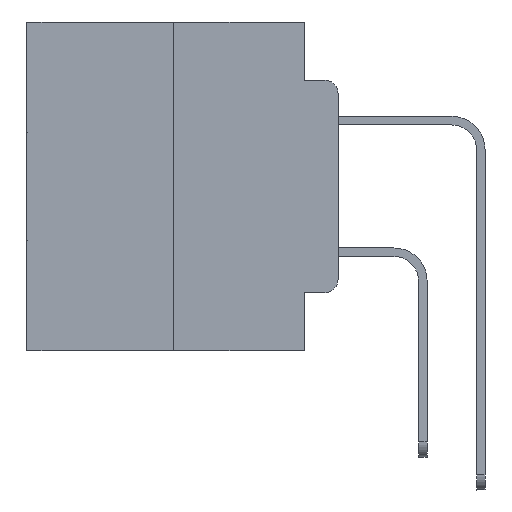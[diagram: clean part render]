
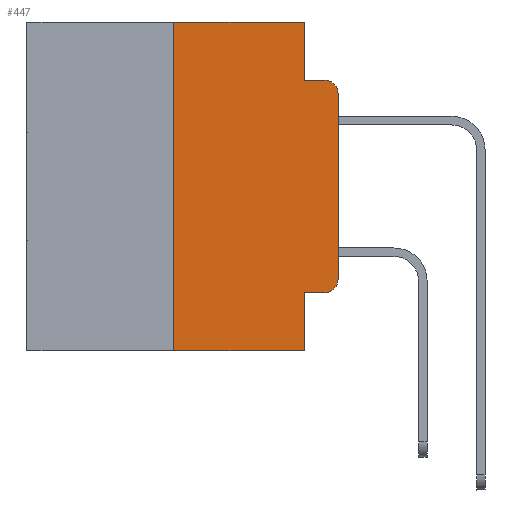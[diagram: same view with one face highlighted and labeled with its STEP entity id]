
A CAD part, left-side view. The second image highlights one B-rep face of the part: STEP entity #447.
In plain terms, the highlighted planar face has unit normal (-1, 0, 0).
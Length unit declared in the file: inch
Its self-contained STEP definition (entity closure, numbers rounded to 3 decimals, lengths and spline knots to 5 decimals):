
#235 = EDGE_CURVE ( 'NONE', #19456, #12653, #22471, .T. ) ;
#362 = VECTOR ( 'NONE', #22300, 39.37008 ) ;
#447 = ADVANCED_FACE ( 'NONE', ( #14925 ), #15079, .F. ) ;
#984 = CARTESIAN_POINT ( 'NONE',  ( 0., 0.02, -0.3915 ) ) ;
#1323 = DIRECTION ( 'NONE',  ( -1., 0., 0. ) ) ;
#1924 = CARTESIAN_POINT ( 'NONE',  ( 0., 0., 0. ) ) ;
#1973 = DIRECTION ( 'NONE',  ( 0., -1., 0. ) ) ;
#2966 = CARTESIAN_POINT ( 'NONE',  ( 0., 0., -0.1085 ) ) ;
#3199 = DIRECTION ( 'NONE',  ( 0., 0., -1. ) ) ;
#3231 = EDGE_CURVE ( 'NONE', #5641, #22865, #3987, .T. ) ;
#3450 = VECTOR ( 'NONE', #3199, 39.37008 ) ;
#3684 = CARTESIAN_POINT ( 'NONE',  ( 0., 0.473, 0. ) ) ;
#3987 = LINE ( 'NONE', #13137, #362 ) ;
#4691 = VECTOR ( 'NONE', #29355, 39.37008 ) ;
#5473 = DIRECTION ( 'NONE',  ( 0., 0., -1. ) ) ;
#5543 = VECTOR ( 'NONE', #1973, 39.37008 ) ;
#5582 = AXIS2_PLACEMENT_3D ( 'NONE', #3684, #28126, #5933 ) ;
#5641 = VERTEX_POINT ( 'NONE', #26946 ) ;
#5727 = CARTESIAN_POINT ( 'NONE',  ( 0., 0.051, -0.0885 ) ) ;
#5933 = DIRECTION ( 'NONE',  ( 0., 0., -1. ) ) ;
#6357 = EDGE_LOOP ( 'NONE', ( #26789, #13331, #10623, #20446, #7698, #7460, #16850, #11954, #8462, #14721 ) ) ;
#6523 = VERTEX_POINT ( 'NONE', #20113 ) ;
#6768 = CIRCLE ( 'NONE', #25910, 0.02 ) ;
#6802 = EDGE_CURVE ( 'NONE', #23607, #6523, #17517, .T. ) ;
#7460 = ORIENTED_EDGE ( 'NONE', *, *, #8773, .F. ) ;
#7513 = CARTESIAN_POINT ( 'NONE',  ( 0., 0., -0.3915 ) ) ;
#7698 = ORIENTED_EDGE ( 'NONE', *, *, #21882, .F. ) ;
#8462 = ORIENTED_EDGE ( 'NONE', *, *, #22431, .T. ) ;
#8677 = CARTESIAN_POINT ( 'NONE',  ( 0., 0.051, -0.5 ) ) ;
#8703 = CARTESIAN_POINT ( 'NONE',  ( 0., 0.051, 0. ) ) ;
#8773 = EDGE_CURVE ( 'NONE', #5641, #13053, #28066, .T. ) ;
#8886 = CARTESIAN_POINT ( 'NONE',  ( 0., 0.473, 0. ) ) ;
#9322 = CARTESIAN_POINT ( 'NONE',  ( 0., 0.051, -0.4115 ) ) ;
#9375 = VECTOR ( 'NONE', #14122, 39.37008 ) ;
#10235 = CARTESIAN_POINT ( 'NONE',  ( 0., 0.051, 0. ) ) ;
#10623 = ORIENTED_EDGE ( 'NONE', *, *, #6802, .F. ) ;
#11954 = ORIENTED_EDGE ( 'NONE', *, *, #19125, .F. ) ;
#12653 = VERTEX_POINT ( 'NONE', #2966 ) ;
#12860 = EDGE_CURVE ( 'NONE', #12653, #6523, #17904, .T. ) ;
#13053 = VERTEX_POINT ( 'NONE', #24551 ) ;
#13137 = CARTESIAN_POINT ( 'NONE',  ( 0., 0.473, -0.5 ) ) ;
#13331 = ORIENTED_EDGE ( 'NONE', *, *, #12860, .T. ) ;
#13591 = AXIS2_PLACEMENT_3D ( 'NONE', #24104, #1323, #19617 ) ;
#13661 = VECTOR ( 'NONE', #27043, 39.37008 ) ;
#14122 = DIRECTION ( 'NONE',  ( 0., 0., 1. ) ) ;
#14721 = ORIENTED_EDGE ( 'NONE', *, *, #27677, .T. ) ;
#14907 = VERTEX_POINT ( 'NONE', #22864 ) ;
#14925 = FACE_OUTER_BOUND ( 'NONE', #6357, .T. ) ;
#15079 = PLANE ( 'NONE',  #5582 ) ;
#15189 = CARTESIAN_POINT ( 'NONE',  ( 0., 0.051, 0. ) ) ;
#15257 = DIRECTION ( 'NONE',  ( 0., -1., 0. ) ) ;
#15433 = VECTOR ( 'NONE', #15257, 39.37008 ) ;
#16850 = ORIENTED_EDGE ( 'NONE', *, *, #3231, .T. ) ;
#17517 = LINE ( 'NONE', #28307, #15433 ) ;
#17904 = CIRCLE ( 'NONE', #13591, 0.02 ) ;
#18778 = CARTESIAN_POINT ( 'NONE',  ( 0., 0.25, 0. ) ) ;
#19103 = LINE ( 'NONE', #10235, #3450 ) ;
#19125 = EDGE_CURVE ( 'NONE', #29437, #22865, #19103, .T. ) ;
#19262 = VERTEX_POINT ( 'NONE', #15189 ) ;
#19456 = VERTEX_POINT ( 'NONE', #7513 ) ;
#19617 = DIRECTION ( 'NONE',  ( 0., 0., -1. ) ) ;
#20113 = CARTESIAN_POINT ( 'NONE',  ( 0., 0.02, -0.0885 ) ) ;
#20446 = ORIENTED_EDGE ( 'NONE', *, *, #21035, .F. ) ;
#21035 = EDGE_CURVE ( 'NONE', #19262, #23607, #29401, .T. ) ;
#21882 = EDGE_CURVE ( 'NONE', #13053, #19262, #27481, .T. ) ;
#22300 = DIRECTION ( 'NONE',  ( 0., -1., 0. ) ) ;
#22431 = EDGE_CURVE ( 'NONE', #29437, #14907, #24755, .T. ) ;
#22471 = LINE ( 'NONE', #1924, #4691 ) ;
#22810 = CARTESIAN_POINT ( 'NONE',  ( 0., 0.051, -0.4115 ) ) ;
#22864 = CARTESIAN_POINT ( 'NONE',  ( 0., 0.02, -0.4115 ) ) ;
#22865 = VERTEX_POINT ( 'NONE', #8677 ) ;
#23607 = VERTEX_POINT ( 'NONE', #5727 ) ;
#23767 = DIRECTION ( 'NONE',  ( -1., 0., 0. ) ) ;
#24104 = CARTESIAN_POINT ( 'NONE',  ( 0., 0.02, -0.1085 ) ) ;
#24463 = DIRECTION ( 'NONE',  ( 0., 0., -1. ) ) ;
#24551 = CARTESIAN_POINT ( 'NONE',  ( 0., 0.25, 0. ) ) ;
#24755 = LINE ( 'NONE', #22810, #5543 ) ;
#25104 = VECTOR ( 'NONE', #24463, 39.37008 ) ;
#25910 = AXIS2_PLACEMENT_3D ( 'NONE', #984, #23767, #5473 ) ;
#26789 = ORIENTED_EDGE ( 'NONE', *, *, #235, .T. ) ;
#26946 = CARTESIAN_POINT ( 'NONE',  ( 0., 0.25, -0.5 ) ) ;
#27043 = DIRECTION ( 'NONE',  ( 0., -1., 0. ) ) ;
#27481 = LINE ( 'NONE', #8886, #13661 ) ;
#27677 = EDGE_CURVE ( 'NONE', #14907, #19456, #6768, .T. ) ;
#28066 = LINE ( 'NONE', #18778, #9375 ) ;
#28126 = DIRECTION ( 'NONE',  ( 1., 0., 0. ) ) ;
#28307 = CARTESIAN_POINT ( 'NONE',  ( 0., 0.051, -0.0885 ) ) ;
#29355 = DIRECTION ( 'NONE',  ( 0., 0., 1. ) ) ;
#29401 = LINE ( 'NONE', #8703, #25104 ) ;
#29437 = VERTEX_POINT ( 'NONE', #9322 ) ;
